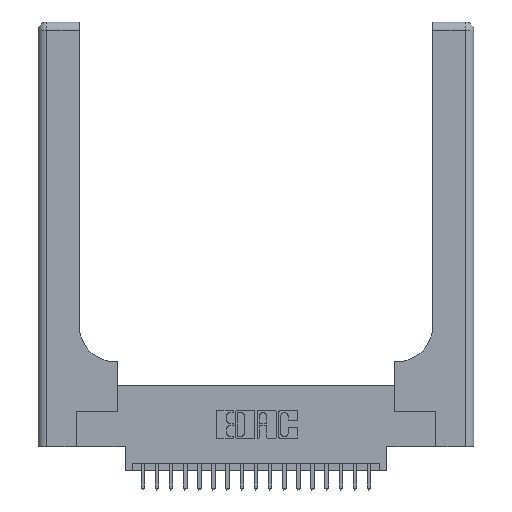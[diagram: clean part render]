
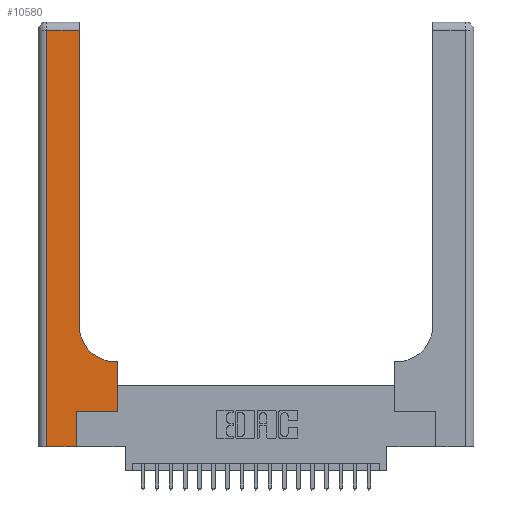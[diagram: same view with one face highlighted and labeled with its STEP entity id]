
A CAD part, top view. The second image highlights one B-rep face of the part: STEP entity #10580.
In plain terms, the highlighted planar face has unit normal (0, 0, 1).
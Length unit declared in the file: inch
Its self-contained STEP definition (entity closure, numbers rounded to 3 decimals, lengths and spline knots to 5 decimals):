
#43 = LINE ( 'NONE', #17762, #17640 ) ;
#220 = DIRECTION ( 'NONE',  ( 0., 1., 0. ) ) ;
#314 = VERTEX_POINT ( 'NONE', #6457 ) ;
#479 = LINE ( 'NONE', #20335, #8761 ) ;
#933 = CARTESIAN_POINT ( 'NONE',  ( 0., 0., 0.37 ) ) ;
#1277 = AXIS2_PLACEMENT_3D ( 'NONE', #10654, #12390, #2153 ) ;
#1440 = VERTEX_POINT ( 'NONE', #19051 ) ;
#1619 = CARTESIAN_POINT ( 'NONE',  ( 0., 3., 0.37 ) ) ;
#2153 = DIRECTION ( 'NONE',  ( 1., 0., 0. ) ) ;
#2294 = PLANE ( 'NONE',  #19618 ) ;
#2685 = CARTESIAN_POINT ( 'NONE',  ( 0.2915, 0.6, 0.37 ) ) ;
#3016 = EDGE_CURVE ( 'NONE', #10416, #12518, #19621, .T. ) ;
#3352 = VERTEX_POINT ( 'NONE', #18743 ) ;
#3374 = LINE ( 'NONE', #17429, #18831 ) ;
#3666 = ORIENTED_EDGE ( 'NONE', *, *, #15531, .T. ) ;
#3830 = EDGE_CURVE ( 'NONE', #17742, #20560, #8650, .T. ) ;
#3847 = DIRECTION ( 'NONE',  ( 0., 0., -1. ) ) ;
#3863 = VECTOR ( 'NONE', #10732, 39.37008 ) ;
#4018 = EDGE_LOOP ( 'NONE', ( #7498, #3666, #16922, #6454, #16312, #14508, #4740, #12875, #14464 ) ) ;
#4740 = ORIENTED_EDGE ( 'NONE', *, *, #3830, .T. ) ;
#6454 = ORIENTED_EDGE ( 'NONE', *, *, #15020, .T. ) ;
#6457 = CARTESIAN_POINT ( 'NONE',  ( 0.2915, 2.94, 0.37 ) ) ;
#6566 = VECTOR ( 'NONE', #18022, 39.37008 ) ;
#7218 = EDGE_CURVE ( 'NONE', #20560, #12677, #15367, .T. ) ;
#7350 = CARTESIAN_POINT ( 'NONE',  ( 0.06, 2.94, 0.37 ) ) ;
#7498 = ORIENTED_EDGE ( 'NONE', *, *, #17057, .T. ) ;
#7703 = CARTESIAN_POINT ( 'NONE',  ( 0.269, 0., 0.37 ) ) ;
#7787 = DIRECTION ( 'NONE',  ( -1., 0., 0. ) ) ;
#8650 = LINE ( 'NONE', #20940, #3863 ) ;
#8761 = VECTOR ( 'NONE', #10050, 39.37008 ) ;
#8852 = EDGE_CURVE ( 'NONE', #12518, #17742, #479, .T. ) ;
#8913 = CARTESIAN_POINT ( 'NONE',  ( 0.5585, 0.25, 0.37 ) ) ;
#9014 = VECTOR ( 'NONE', #220, 39.37008 ) ;
#9593 = VECTOR ( 'NONE', #12890, 39.37008 ) ;
#10050 = DIRECTION ( 'NONE',  ( 1., 0., 0. ) ) ;
#10285 = FACE_OUTER_BOUND ( 'NONE', #4018, .T. ) ;
#10416 = VERTEX_POINT ( 'NONE', #7703 ) ;
#10580 = ADVANCED_FACE ( 'NONE', ( #10285 ), #2294, .F. ) ;
#10640 = LINE ( 'NONE', #933, #9593 ) ;
#10654 = CARTESIAN_POINT ( 'NONE',  ( 0.5415, 0.85, 0.37 ) ) ;
#10732 = DIRECTION ( 'NONE',  ( 0., 1., 0. ) ) ;
#11333 = VERTEX_POINT ( 'NONE', #7350 ) ;
#12169 = VECTOR ( 'NONE', #7787, 39.37008 ) ;
#12390 = DIRECTION ( 'NONE',  ( 0., 0., -1. ) ) ;
#12392 = DIRECTION ( 'NONE',  ( -1., 0., 0. ) ) ;
#12518 = VERTEX_POINT ( 'NONE', #18969 ) ;
#12578 = EDGE_CURVE ( 'NONE', #11333, #1440, #43, .T. ) ;
#12677 = VERTEX_POINT ( 'NONE', #13367 ) ;
#12684 = CARTESIAN_POINT ( 'NONE',  ( 0.5585, 0.6, 0.37 ) ) ;
#12875 = ORIENTED_EDGE ( 'NONE', *, *, #7218, .T. ) ;
#12890 = DIRECTION ( 'NONE',  ( 1., 0., 0. ) ) ;
#13367 = CARTESIAN_POINT ( 'NONE',  ( 0.5415, 0.6, 0.37 ) ) ;
#13573 = LINE ( 'NONE', #18723, #9014 ) ;
#13816 = CIRCLE ( 'NONE', #1277, 0.25 ) ;
#14464 = ORIENTED_EDGE ( 'NONE', *, *, #17126, .T. ) ;
#14508 = ORIENTED_EDGE ( 'NONE', *, *, #8852, .T. ) ;
#15020 = EDGE_CURVE ( 'NONE', #1440, #10416, #10640, .T. ) ;
#15367 = LINE ( 'NONE', #2685, #12169 ) ;
#15531 = EDGE_CURVE ( 'NONE', #314, #11333, #3374, .T. ) ;
#15785 = DIRECTION ( 'NONE',  ( -1., 0., 0. ) ) ;
#16312 = ORIENTED_EDGE ( 'NONE', *, *, #3016, .T. ) ;
#16922 = ORIENTED_EDGE ( 'NONE', *, *, #12578, .T. ) ;
#17057 = EDGE_CURVE ( 'NONE', #3352, #314, #13573, .T. ) ;
#17126 = EDGE_CURVE ( 'NONE', #12677, #3352, #13816, .T. ) ;
#17429 = CARTESIAN_POINT ( 'NONE',  ( 0., 2.94, 0.37 ) ) ;
#17640 = VECTOR ( 'NONE', #21261, 39.37008 ) ;
#17742 = VERTEX_POINT ( 'NONE', #8913 ) ;
#17762 = CARTESIAN_POINT ( 'NONE',  ( 0.06, 3., 0.37 ) ) ;
#18022 = DIRECTION ( 'NONE',  ( 0., 1., 0. ) ) ;
#18723 = CARTESIAN_POINT ( 'NONE',  ( 0.2915, 3., 0.37 ) ) ;
#18743 = CARTESIAN_POINT ( 'NONE',  ( 0.2915, 0.85, 0.37 ) ) ;
#18831 = VECTOR ( 'NONE', #12392, 39.37008 ) ;
#18969 = CARTESIAN_POINT ( 'NONE',  ( 0.269, 0.25, 0.37 ) ) ;
#19051 = CARTESIAN_POINT ( 'NONE',  ( 0.06, 0., 0.37 ) ) ;
#19618 = AXIS2_PLACEMENT_3D ( 'NONE', #1619, #3847, #15785 ) ;
#19621 = LINE ( 'NONE', #19880, #6566 ) ;
#19880 = CARTESIAN_POINT ( 'NONE',  ( 0.269, 0., 0.37 ) ) ;
#20335 = CARTESIAN_POINT ( 'NONE',  ( 0.269, 0.25, 0.37 ) ) ;
#20560 = VERTEX_POINT ( 'NONE', #12684 ) ;
#20940 = CARTESIAN_POINT ( 'NONE',  ( 0.5585, 0.25, 0.37 ) ) ;
#21261 = DIRECTION ( 'NONE',  ( 0., -1., 0. ) ) ;
